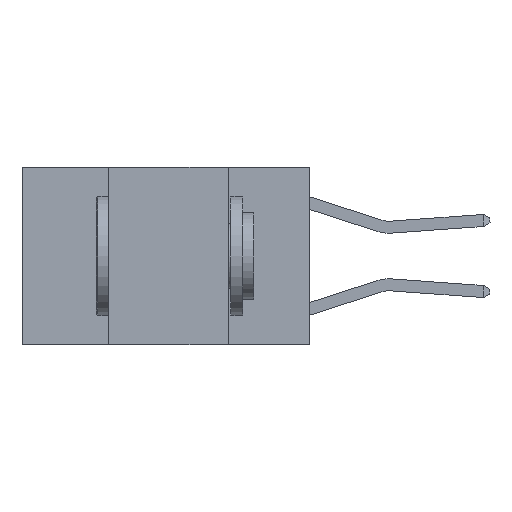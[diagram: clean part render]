
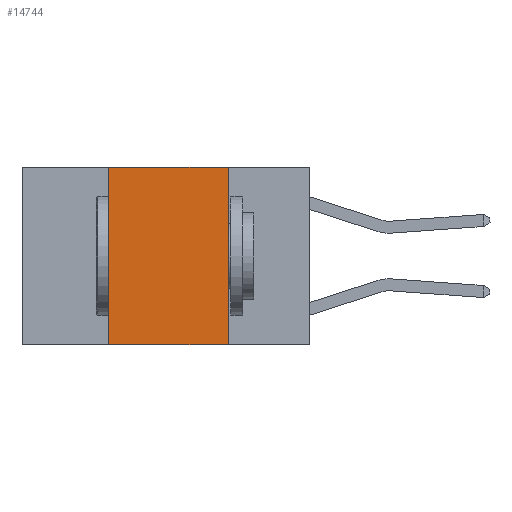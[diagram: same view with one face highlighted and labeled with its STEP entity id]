
A CAD part, left-side view. The second image highlights one B-rep face of the part: STEP entity #14744.
In plain terms, the highlighted planar face has unit normal (-1, 0, 0).
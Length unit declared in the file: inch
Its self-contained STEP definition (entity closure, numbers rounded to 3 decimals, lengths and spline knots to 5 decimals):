
#542 = CARTESIAN_POINT ( 'NONE',  ( 0., 0.6, -0.37 ) ) ;
#2222 = DIRECTION ( 'NONE',  ( 0., 0., 1. ) ) ;
#2620 = CARTESIAN_POINT ( 'NONE',  ( 0., 0.17, 0. ) ) ;
#2995 = VECTOR ( 'NONE', #10728, 39.37008 ) ;
#4849 = EDGE_CURVE ( 'NONE', #13835, #21302, #5570, .T. ) ;
#5570 = LINE ( 'NONE', #6549, #2995 ) ;
#6549 = CARTESIAN_POINT ( 'NONE',  ( 0., 0.6, 0. ) ) ;
#8106 = FACE_OUTER_BOUND ( 'NONE', #24549, .T. ) ;
#8492 = LINE ( 'NONE', #22137, #23024 ) ;
#8588 = EDGE_CURVE ( 'NONE', #24445, #23601, #24908, .T. ) ;
#9214 = LINE ( 'NONE', #2620, #14567 ) ;
#9775 = DIRECTION ( 'NONE',  ( 0., 0., -1. ) ) ;
#10728 = DIRECTION ( 'NONE',  ( 0., -1., 0. ) ) ;
#11729 = PLANE ( 'NONE',  #14441 ) ;
#13384 = ORIENTED_EDGE ( 'NONE', *, *, #4849, .F. ) ;
#13640 = EDGE_CURVE ( 'NONE', #24445, #13835, #8492, .T. ) ;
#13835 = VERTEX_POINT ( 'NONE', #24646 ) ;
#14441 = AXIS2_PLACEMENT_3D ( 'NONE', #19648, #21641, #9775 ) ;
#14567 = VECTOR ( 'NONE', #22617, 39.37008 ) ;
#14744 = ADVANCED_FACE ( 'NONE', ( #8106 ), #11729, .F. ) ;
#15475 = ORIENTED_EDGE ( 'NONE', *, *, #22494, .F. ) ;
#19648 = CARTESIAN_POINT ( 'NONE',  ( 0., 0.6, 0. ) ) ;
#19810 = CARTESIAN_POINT ( 'NONE',  ( 0., 0.17, -0.37 ) ) ;
#20374 = VECTOR ( 'NONE', #22453, 39.37008 ) ;
#20546 = CARTESIAN_POINT ( 'NONE',  ( 0., 0.42, -0.37 ) ) ;
#21302 = VERTEX_POINT ( 'NONE', #23071 ) ;
#21641 = DIRECTION ( 'NONE',  ( 1., 0., 0. ) ) ;
#22137 = CARTESIAN_POINT ( 'NONE',  ( 0., 0.42, 0. ) ) ;
#22262 = ORIENTED_EDGE ( 'NONE', *, *, #8588, .T. ) ;
#22453 = DIRECTION ( 'NONE',  ( 0., -1., 0. ) ) ;
#22494 = EDGE_CURVE ( 'NONE', #21302, #23601, #9214, .T. ) ;
#22617 = DIRECTION ( 'NONE',  ( 0., 0., -1. ) ) ;
#23024 = VECTOR ( 'NONE', #2222, 39.37008 ) ;
#23071 = CARTESIAN_POINT ( 'NONE',  ( 0., 0.17, 0. ) ) ;
#23601 = VERTEX_POINT ( 'NONE', #19810 ) ;
#23666 = ORIENTED_EDGE ( 'NONE', *, *, #13640, .F. ) ;
#24445 = VERTEX_POINT ( 'NONE', #20546 ) ;
#24549 = EDGE_LOOP ( 'NONE', ( #15475, #13384, #23666, #22262 ) ) ;
#24646 = CARTESIAN_POINT ( 'NONE',  ( 0., 0.42, 0. ) ) ;
#24908 = LINE ( 'NONE', #542, #20374 ) ;
